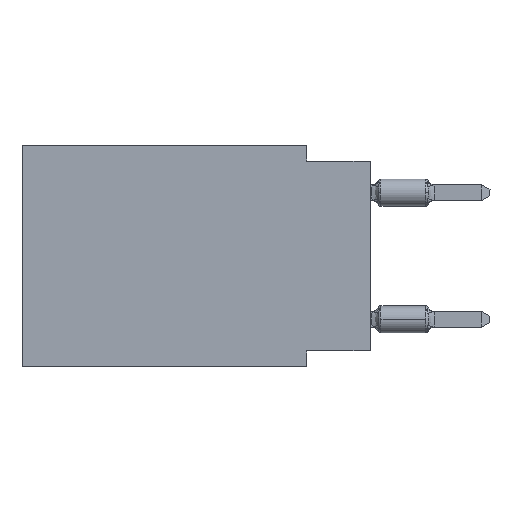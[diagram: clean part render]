
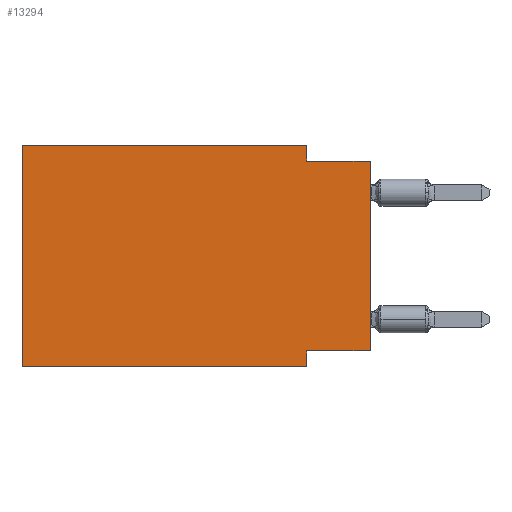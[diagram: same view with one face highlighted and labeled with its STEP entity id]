
A CAD part, left-side view. The second image highlights one B-rep face of the part: STEP entity #13294.
In plain terms, the highlighted planar face has unit normal (-1, 0, 0).
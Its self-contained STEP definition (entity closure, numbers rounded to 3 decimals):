
#66 = DIRECTION ( 'NONE',  ( 0., 0., 1. ) ) ;
#436 = DIRECTION ( 'NONE',  ( 0., 0., 1. ) ) ;
#499 = VERTEX_POINT ( 'NONE', #2474 ) ;
#540 = VERTEX_POINT ( 'NONE', #9007 ) ;
#779 = CARTESIAN_POINT ( 'NONE',  ( 0., 13.97, 0. ) ) ;
#846 = ORIENTED_EDGE ( 'NONE', *, *, #9660, .T. ) ;
#868 = VECTOR ( 'NONE', #12378, 1000. ) ;
#941 = EDGE_CURVE ( 'NONE', #6902, #540, #2012, .T. ) ;
#1186 = VECTOR ( 'NONE', #436, 1000. ) ;
#1283 = LINE ( 'NONE', #9651, #4132 ) ;
#1287 = ORIENTED_EDGE ( 'NONE', *, *, #941, .F. ) ;
#1367 = VERTEX_POINT ( 'NONE', #5090 ) ;
#1574 = CARTESIAN_POINT ( 'NONE',  ( 0., 0., -0.635 ) ) ;
#1788 = DIRECTION ( 'NONE',  ( 0., 0., -1. ) ) ;
#2012 = LINE ( 'NONE', #6212, #868 ) ;
#2026 = VECTOR ( 'NONE', #2958, 1000. ) ;
#2438 = ORIENTED_EDGE ( 'NONE', *, *, #12972, .F. ) ;
#2474 = CARTESIAN_POINT ( 'NONE',  ( 0., 13.97, -8.89 ) ) ;
#2958 = DIRECTION ( 'NONE',  ( 0., 0., -1. ) ) ;
#3614 = EDGE_CURVE ( 'NONE', #11541, #10486, #13324, .T. ) ;
#4122 = CARTESIAN_POINT ( 'NONE',  ( 0., 2.54, -8.89 ) ) ;
#4132 = VECTOR ( 'NONE', #13577, 1000. ) ;
#4826 = VECTOR ( 'NONE', #66, 1000. ) ;
#4986 = DIRECTION ( 'NONE',  ( 0., 0., -1. ) ) ;
#5023 = VECTOR ( 'NONE', #10703, 1000. ) ;
#5090 = CARTESIAN_POINT ( 'NONE',  ( 0., 13.97, 0. ) ) ;
#5576 = EDGE_LOOP ( 'NONE', ( #846, #2438, #12721, #10125, #7145, #12422, #7158, #1287 ) ) ;
#5662 = VERTEX_POINT ( 'NONE', #1574 ) ;
#5919 = CARTESIAN_POINT ( 'NONE',  ( 0., 2.54, -8.89 ) ) ;
#5936 = EDGE_CURVE ( 'NONE', #499, #1367, #9839, .T. ) ;
#6052 = LINE ( 'NONE', #4122, #8696 ) ;
#6212 = CARTESIAN_POINT ( 'NONE',  ( 0., 0., -8.255 ) ) ;
#6902 = VERTEX_POINT ( 'NONE', #8313 ) ;
#7145 = ORIENTED_EDGE ( 'NONE', *, *, #5936, .F. ) ;
#7158 = ORIENTED_EDGE ( 'NONE', *, *, #11074, .F. ) ;
#7256 = EDGE_CURVE ( 'NONE', #1367, #11541, #9045, .T. ) ;
#8235 = CARTESIAN_POINT ( 'NONE',  ( 0., 2.54, 0. ) ) ;
#8283 = DIRECTION ( 'NONE',  ( 1., 0., 0. ) ) ;
#8313 = CARTESIAN_POINT ( 'NONE',  ( 0., 0., -8.255 ) ) ;
#8661 = LINE ( 'NONE', #9485, #4826 ) ;
#8696 = VECTOR ( 'NONE', #1788, 1000. ) ;
#9007 = CARTESIAN_POINT ( 'NONE',  ( 0., 2.54, -8.255 ) ) ;
#9045 = LINE ( 'NONE', #13094, #11071 ) ;
#9404 = AXIS2_PLACEMENT_3D ( 'NONE', #779, #8283, #4986 ) ;
#9485 = CARTESIAN_POINT ( 'NONE',  ( 0., 0., 0. ) ) ;
#9651 = CARTESIAN_POINT ( 'NONE',  ( 0., 0., -0.635 ) ) ;
#9660 = EDGE_CURVE ( 'NONE', #6902, #5662, #8661, .T. ) ;
#9839 = LINE ( 'NONE', #11848, #1186 ) ;
#10125 = ORIENTED_EDGE ( 'NONE', *, *, #7256, .F. ) ;
#10187 = PLANE ( 'NONE',  #9404 ) ;
#10486 = VERTEX_POINT ( 'NONE', #11965 ) ;
#10703 = DIRECTION ( 'NONE',  ( 0., -1., 0. ) ) ;
#10968 = DIRECTION ( 'NONE',  ( 0., -1., 0. ) ) ;
#11071 = VECTOR ( 'NONE', #10968, 1000. ) ;
#11074 = EDGE_CURVE ( 'NONE', #540, #12336, #6052, .T. ) ;
#11228 = FACE_OUTER_BOUND ( 'NONE', #5576, .T. ) ;
#11534 = CARTESIAN_POINT ( 'NONE',  ( 0., 13.97, -8.89 ) ) ;
#11541 = VERTEX_POINT ( 'NONE', #8235 ) ;
#11848 = CARTESIAN_POINT ( 'NONE',  ( 0., 13.97, 0. ) ) ;
#11965 = CARTESIAN_POINT ( 'NONE',  ( 0., 2.54, -0.635 ) ) ;
#12336 = VERTEX_POINT ( 'NONE', #5919 ) ;
#12378 = DIRECTION ( 'NONE',  ( 0., 1., 0. ) ) ;
#12422 = ORIENTED_EDGE ( 'NONE', *, *, #12595, .T. ) ;
#12595 = EDGE_CURVE ( 'NONE', #499, #12336, #12826, .T. ) ;
#12721 = ORIENTED_EDGE ( 'NONE', *, *, #3614, .F. ) ;
#12826 = LINE ( 'NONE', #11534, #5023 ) ;
#12972 = EDGE_CURVE ( 'NONE', #10486, #5662, #1283, .T. ) ;
#13094 = CARTESIAN_POINT ( 'NONE',  ( 0., 13.97, 0. ) ) ;
#13294 = ADVANCED_FACE ( 'NONE', ( #11228 ), #10187, .F. ) ;
#13324 = LINE ( 'NONE', #13390, #2026 ) ;
#13390 = CARTESIAN_POINT ( 'NONE',  ( 0., 2.54, 0. ) ) ;
#13577 = DIRECTION ( 'NONE',  ( 0., -1., 0. ) ) ;
